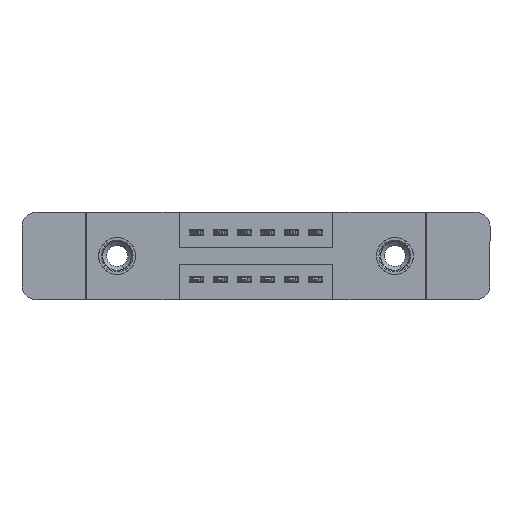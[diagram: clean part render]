
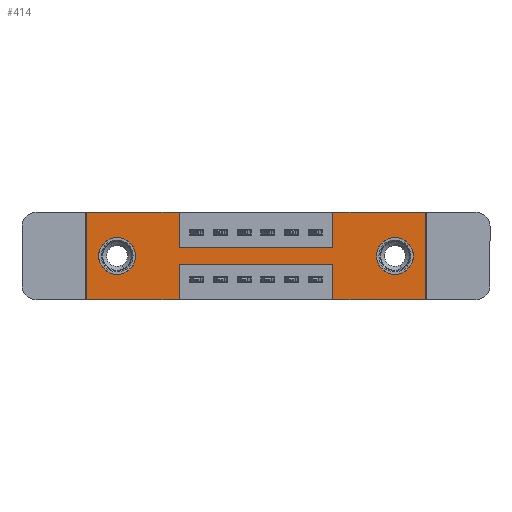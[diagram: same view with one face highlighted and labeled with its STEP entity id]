
A CAD part, front view. The second image highlights one B-rep face of the part: STEP entity #414.
In plain terms, the highlighted planar face has unit normal (0, -1, 0).
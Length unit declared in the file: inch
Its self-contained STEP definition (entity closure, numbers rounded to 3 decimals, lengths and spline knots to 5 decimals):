
#293 = CARTESIAN_POINT ( 'NONE',  ( 1.305, 0., -0.185 ) ) ;
#414 = ADVANCED_FACE ( 'NONE', ( #836, #11067, #9680 ), #7712, .T. ) ;
#494 = VERTEX_POINT ( 'NONE', #12337 ) ;
#534 = VECTOR ( 'NONE', #9279, 39.37008 ) ;
#567 = CARTESIAN_POINT ( 'NONE',  ( 0., 0., -0.37 ) ) ;
#601 = DIRECTION ( 'NONE',  ( 0., 0., 1. ) ) ;
#616 = DIRECTION ( 'NONE',  ( -1., 0., 0. ) ) ;
#773 = VECTOR ( 'NONE', #9138, 39.37008 ) ;
#824 = ORIENTED_EDGE ( 'NONE', *, *, #7998, .F. ) ;
#836 = FACE_BOUND ( 'NONE', #13256, .T. ) ;
#838 = LINE ( 'NONE', #4488, #6615 ) ;
#922 = ORIENTED_EDGE ( 'NONE', *, *, #14004, .T. ) ;
#994 = CARTESIAN_POINT ( 'NONE',  ( 0.13, 0., -0.263 ) ) ;
#1082 = EDGE_CURVE ( 'NONE', #7855, #9353, #4126, .T. ) ;
#1133 = CARTESIAN_POINT ( 'NONE',  ( 0.13, 0., -0.185 ) ) ;
#1295 = CARTESIAN_POINT ( 'NONE',  ( 0.3925, 0., -0.15 ) ) ;
#1315 = CARTESIAN_POINT ( 'NONE',  ( 0.13, 0., -0.185 ) ) ;
#1318 = ORIENTED_EDGE ( 'NONE', *, *, #3305, .T. ) ;
#1676 = ORIENTED_EDGE ( 'NONE', *, *, #5050, .F. ) ;
#1951 = DIRECTION ( 'NONE',  ( 0., 0., -1. ) ) ;
#1958 = DIRECTION ( 'NONE',  ( 0., 1., 0. ) ) ;
#2121 = ORIENTED_EDGE ( 'NONE', *, *, #1082, .F. ) ;
#2242 = CARTESIAN_POINT ( 'NONE',  ( 0.3925, 0., -0.15 ) ) ;
#2259 = CARTESIAN_POINT ( 'NONE',  ( 1.0425, 0., -0.22 ) ) ;
#2283 = DIRECTION ( 'NONE',  ( 0., 0., 1. ) ) ;
#2522 = VERTEX_POINT ( 'NONE', #2839 ) ;
#2536 = DIRECTION ( 'NONE',  ( -1., 0., 0. ) ) ;
#2615 = CIRCLE ( 'NONE', #3074, 0.078 ) ;
#2617 = LINE ( 'NONE', #9606, #12291 ) ;
#2783 = EDGE_CURVE ( 'NONE', #11576, #5616, #8091, .T. ) ;
#2839 = CARTESIAN_POINT ( 'NONE',  ( 0., 0., -0.37 ) ) ;
#2883 = ORIENTED_EDGE ( 'NONE', *, *, #6117, .F. ) ;
#3074 = AXIS2_PLACEMENT_3D ( 'NONE', #10023, #1958, #12202 ) ;
#3279 = EDGE_CURVE ( 'NONE', #11008, #9819, #5873, .T. ) ;
#3305 = EDGE_CURVE ( 'NONE', #3824, #8897, #2615, .T. ) ;
#3483 = CARTESIAN_POINT ( 'NONE',  ( 0.3925, 0., 0. ) ) ;
#3651 = LINE ( 'NONE', #8594, #10444 ) ;
#3701 = VERTEX_POINT ( 'NONE', #10735 ) ;
#3824 = VERTEX_POINT ( 'NONE', #9855 ) ;
#3856 = VERTEX_POINT ( 'NONE', #5137 ) ;
#3925 = CARTESIAN_POINT ( 'NONE',  ( 0.3925, 0., -0.37 ) ) ;
#4105 = CARTESIAN_POINT ( 'NONE',  ( 0.13, 0., -0.107 ) ) ;
#4126 = LINE ( 'NONE', #3925, #11836 ) ;
#4134 = EDGE_CURVE ( 'NONE', #10120, #11576, #7569, .T. ) ;
#4191 = ORIENTED_EDGE ( 'NONE', *, *, #3279, .T. ) ;
#4471 = VECTOR ( 'NONE', #2283, 39.37008 ) ;
#4488 = CARTESIAN_POINT ( 'NONE',  ( 0., 0., 0. ) ) ;
#4530 = EDGE_CURVE ( 'NONE', #8174, #7036, #13645, .T. ) ;
#4555 = CARTESIAN_POINT ( 'NONE',  ( 1.0425, 0., -0.37 ) ) ;
#4843 = DIRECTION ( 'NONE',  ( 0., 0., 1. ) ) ;
#4884 = VERTEX_POINT ( 'NONE', #14296 ) ;
#5050 = EDGE_CURVE ( 'NONE', #7036, #7855, #11289, .T. ) ;
#5137 = CARTESIAN_POINT ( 'NONE',  ( 0.3925, 0., 0. ) ) ;
#5408 = CARTESIAN_POINT ( 'NONE',  ( 0.3925, 0., -0.37 ) ) ;
#5570 = CARTESIAN_POINT ( 'NONE',  ( 0.3925, 0., -0.22 ) ) ;
#5612 = CARTESIAN_POINT ( 'NONE',  ( 1.305, 0., -0.107 ) ) ;
#5616 = VERTEX_POINT ( 'NONE', #13572 ) ;
#5629 = ORIENTED_EDGE ( 'NONE', *, *, #13889, .F. ) ;
#5689 = DIRECTION ( 'NONE',  ( 0., 0., 1. ) ) ;
#5873 = CIRCLE ( 'NONE', #7297, 0.078 ) ;
#6019 = EDGE_CURVE ( 'NONE', #5616, #4884, #7002, .T. ) ;
#6100 = ORIENTED_EDGE ( 'NONE', *, *, #4530, .F. ) ;
#6117 = EDGE_CURVE ( 'NONE', #3701, #3856, #838, .T. ) ;
#6172 = DIRECTION ( 'NONE',  ( 0., 0., -1. ) ) ;
#6615 = VECTOR ( 'NONE', #8078, 39.37008 ) ;
#6929 = LINE ( 'NONE', #3483, #773 ) ;
#7002 = LINE ( 'NONE', #14555, #11068 ) ;
#7036 = VERTEX_POINT ( 'NONE', #2259 ) ;
#7103 = CARTESIAN_POINT ( 'NONE',  ( 1.0425, 0., 0. ) ) ;
#7185 = EDGE_CURVE ( 'NONE', #9819, #11008, #11767, .T. ) ;
#7297 = AXIS2_PLACEMENT_3D ( 'NONE', #1133, #10272, #9201 ) ;
#7306 = ORIENTED_EDGE ( 'NONE', *, *, #7185, .T. ) ;
#7536 = VECTOR ( 'NONE', #8020, 39.37008 ) ;
#7569 = LINE ( 'NONE', #2242, #534 ) ;
#7574 = CARTESIAN_POINT ( 'NONE',  ( 0.3925, 0., -0.22 ) ) ;
#7712 = PLANE ( 'NONE',  #13723 ) ;
#7768 = VECTOR ( 'NONE', #9666, 39.37008 ) ;
#7787 = ORIENTED_EDGE ( 'NONE', *, *, #13359, .F. ) ;
#7855 = VERTEX_POINT ( 'NONE', #7574 ) ;
#7986 = ORIENTED_EDGE ( 'NONE', *, *, #2783, .F. ) ;
#7998 = EDGE_CURVE ( 'NONE', #9353, #2522, #2617, .T. ) ;
#8020 = DIRECTION ( 'NONE',  ( -1., 0., 0. ) ) ;
#8078 = DIRECTION ( 'NONE',  ( 1., 0., 0. ) ) ;
#8091 = LINE ( 'NONE', #7103, #4471 ) ;
#8132 = DIRECTION ( 'NONE',  ( 0., 1., 0. ) ) ;
#8174 = VERTEX_POINT ( 'NONE', #10950 ) ;
#8513 = CARTESIAN_POINT ( 'NONE',  ( 1.435, 0., 0. ) ) ;
#8541 = ORIENTED_EDGE ( 'NONE', *, *, #4134, .F. ) ;
#8594 = CARTESIAN_POINT ( 'NONE',  ( 0., 0., 0. ) ) ;
#8597 = ORIENTED_EDGE ( 'NONE', *, *, #10261, .F. ) ;
#8696 = LINE ( 'NONE', #8513, #7768 ) ;
#8897 = VERTEX_POINT ( 'NONE', #5612 ) ;
#9004 = AXIS2_PLACEMENT_3D ( 'NONE', #1315, #8132, #4843 ) ;
#9034 = EDGE_CURVE ( 'NONE', #3856, #10120, #6929, .T. ) ;
#9054 = VECTOR ( 'NONE', #616, 39.37008 ) ;
#9138 = DIRECTION ( 'NONE',  ( 0., 0., -1. ) ) ;
#9201 = DIRECTION ( 'NONE',  ( 0., 0., 1. ) ) ;
#9279 = DIRECTION ( 'NONE',  ( 1., 0., 0. ) ) ;
#9353 = VERTEX_POINT ( 'NONE', #5408 ) ;
#9424 = LINE ( 'NONE', #567, #9054 ) ;
#9606 = CARTESIAN_POINT ( 'NONE',  ( 0., 0., -0.37 ) ) ;
#9657 = DIRECTION ( 'NONE',  ( 0., 1., 0. ) ) ;
#9666 = DIRECTION ( 'NONE',  ( 0., 0., -1. ) ) ;
#9680 = FACE_OUTER_BOUND ( 'NONE', #11958, .T. ) ;
#9819 = VERTEX_POINT ( 'NONE', #994 ) ;
#9855 = CARTESIAN_POINT ( 'NONE',  ( 1.305, 0., -0.263 ) ) ;
#10023 = CARTESIAN_POINT ( 'NONE',  ( 1.305, 0., -0.185 ) ) ;
#10120 = VERTEX_POINT ( 'NONE', #1295 ) ;
#10261 = EDGE_CURVE ( 'NONE', #494, #8174, #9424, .T. ) ;
#10272 = DIRECTION ( 'NONE',  ( 0., 1., 0. ) ) ;
#10444 = VECTOR ( 'NONE', #601, 39.37008 ) ;
#10593 = VECTOR ( 'NONE', #5689, 39.37008 ) ;
#10735 = CARTESIAN_POINT ( 'NONE',  ( 0., 0., 0. ) ) ;
#10742 = DIRECTION ( 'NONE',  ( 0., 0., -1. ) ) ;
#10950 = CARTESIAN_POINT ( 'NONE',  ( 1.0425, 0., -0.37 ) ) ;
#11008 = VERTEX_POINT ( 'NONE', #4105 ) ;
#11067 = FACE_BOUND ( 'NONE', #12911, .T. ) ;
#11068 = VECTOR ( 'NONE', #13494, 39.37008 ) ;
#11279 = ORIENTED_EDGE ( 'NONE', *, *, #9034, .F. ) ;
#11289 = LINE ( 'NONE', #5570, #7536 ) ;
#11576 = VERTEX_POINT ( 'NONE', #14115 ) ;
#11767 = CIRCLE ( 'NONE', #9004, 0.078 ) ;
#11836 = VECTOR ( 'NONE', #10742, 39.37008 ) ;
#11958 = EDGE_LOOP ( 'NONE', ( #2121, #1676, #6100, #8597, #7787, #14600, #7986, #8541, #11279, #2883, #5629, #824 ) ) ;
#12202 = DIRECTION ( 'NONE',  ( 0., 0., -1. ) ) ;
#12291 = VECTOR ( 'NONE', #2536, 39.37008 ) ;
#12337 = CARTESIAN_POINT ( 'NONE',  ( 1.435, 0., -0.37 ) ) ;
#12383 = CARTESIAN_POINT ( 'NONE',  ( 0., 0., -0.37 ) ) ;
#12911 = EDGE_LOOP ( 'NONE', ( #4191, #7306 ) ) ;
#12914 = AXIS2_PLACEMENT_3D ( 'NONE', #293, #9657, #6172 ) ;
#13256 = EDGE_LOOP ( 'NONE', ( #922, #1318 ) ) ;
#13359 = EDGE_CURVE ( 'NONE', #4884, #494, #8696, .T. ) ;
#13446 = DIRECTION ( 'NONE',  ( 0., -1., 0. ) ) ;
#13494 = DIRECTION ( 'NONE',  ( 1., 0., 0. ) ) ;
#13572 = CARTESIAN_POINT ( 'NONE',  ( 1.0425, 0., 0. ) ) ;
#13645 = LINE ( 'NONE', #4555, #10593 ) ;
#13723 = AXIS2_PLACEMENT_3D ( 'NONE', #12383, #13446, #1951 ) ;
#13889 = EDGE_CURVE ( 'NONE', #2522, #3701, #3651, .T. ) ;
#14004 = EDGE_CURVE ( 'NONE', #8897, #3824, #14758, .T. ) ;
#14115 = CARTESIAN_POINT ( 'NONE',  ( 1.0425, 0., -0.15 ) ) ;
#14296 = CARTESIAN_POINT ( 'NONE',  ( 1.435, 0., 0. ) ) ;
#14555 = CARTESIAN_POINT ( 'NONE',  ( 0., 0., 0. ) ) ;
#14600 = ORIENTED_EDGE ( 'NONE', *, *, #6019, .F. ) ;
#14758 = CIRCLE ( 'NONE', #12914, 0.078 ) ;
